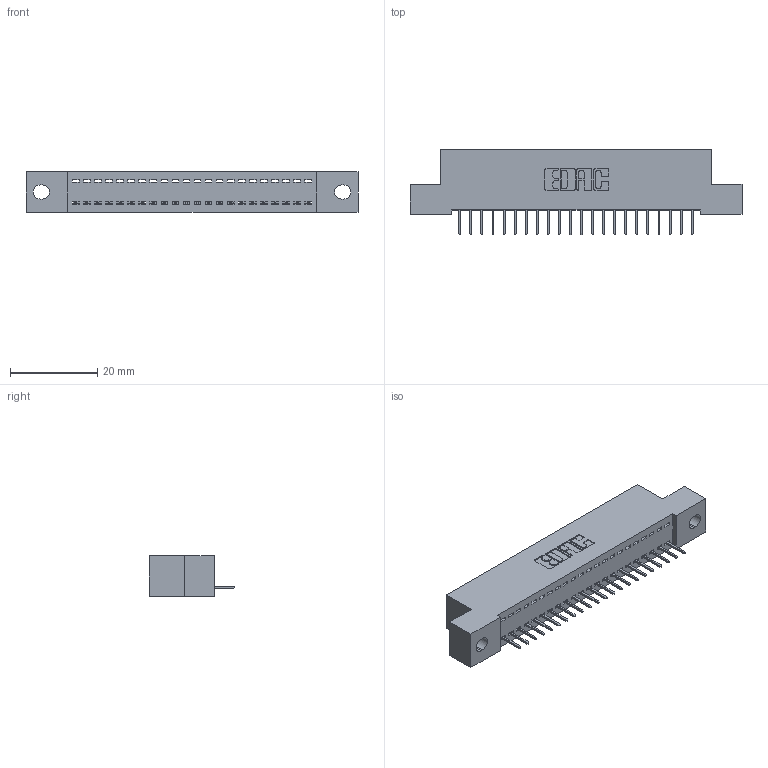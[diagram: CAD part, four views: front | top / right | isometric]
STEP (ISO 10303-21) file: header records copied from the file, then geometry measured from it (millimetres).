
FILE_DESCRIPTION (( 'STEP AP203' ), '1' );
FILE_NAME ('342-022-524-102.STEP', '2019-10-01T22:19:52', ( '' ), ( '' ), 'SwSTEP 2.0', 'SolidWorks 2016', '' );
FILE_SCHEMA (( 'CONFIG_CONTROL_DESIGN' ));
Length unit declared in the file: inch
Products named in the file (3): 345-292-001_345-293-124; 342-022-524-102; 342 Part_.128 Slot
Assembly tree (23 placements, depth 2):
  342-022-524-102
    342 Part_.128 Slot
    345-292-001_345-293-124  x22
Bounding box: 76.2 x 19.69 x 9.4 mm (x, y, z)
Volume: 6468.5 mm3; surface area: 8615 mm2
Topology: 23 solids, 23 shells, 1478 faces, 4271 edges, 2758 vertices
Faces by surface type: plane 1126, cylinder 352
Entity records: 16113 total; most frequent: CARTESIAN_POINT 2788, ORIENTED_EDGE 2746, DIRECTION 2393, EDGE_CURVE 1373, VECTOR 1249, LINE 1249, VERTEX_POINT 910, AXIS2_PLACEMENT_3D 572
